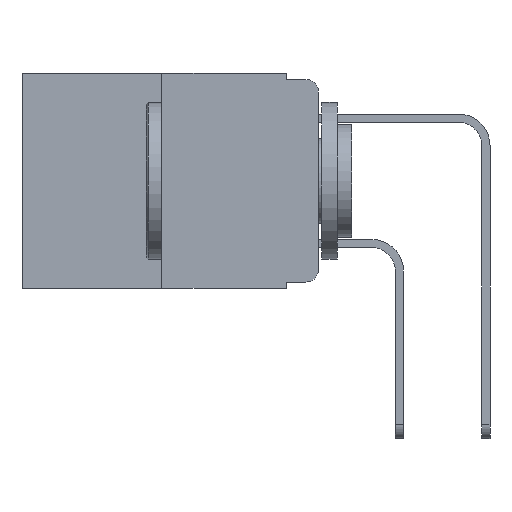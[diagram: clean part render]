
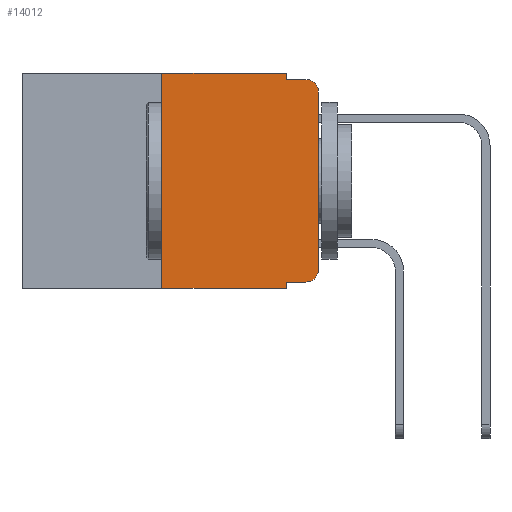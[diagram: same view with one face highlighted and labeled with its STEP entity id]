
A CAD part, left-side view. The second image highlights one B-rep face of the part: STEP entity #14012.
In plain terms, the highlighted planar face has unit normal (-1, 0, 0).
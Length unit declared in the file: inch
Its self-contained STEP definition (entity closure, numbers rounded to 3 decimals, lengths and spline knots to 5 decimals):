
#53 = DIRECTION ( 'NONE',  ( 0., -1., 0. ) ) ;
#161 = ORIENTED_EDGE ( 'NONE', *, *, #11742, .T. ) ;
#222 = VECTOR ( 'NONE', #8040, 39.37008 ) ;
#351 = CARTESIAN_POINT ( 'NONE',  ( 0., 0.051, -0.333 ) ) ;
#518 = ORIENTED_EDGE ( 'NONE', *, *, #749, .T. ) ;
#694 = ORIENTED_EDGE ( 'NONE', *, *, #9672, .F. ) ;
#749 = EDGE_CURVE ( 'NONE', #13618, #11591, #5216, .T. ) ;
#803 = CARTESIAN_POINT ( 'NONE',  ( 0., 0.02, -0.01 ) ) ;
#817 = CARTESIAN_POINT ( 'NONE',  ( 0., 0.473, 0. ) ) ;
#827 = CARTESIAN_POINT ( 'NONE',  ( 0., 0.25, 0. ) ) ;
#982 = VERTEX_POINT ( 'NONE', #7547 ) ;
#1018 = CARTESIAN_POINT ( 'NONE',  ( 0., 0.02, -0.333 ) ) ;
#1307 = VERTEX_POINT ( 'NONE', #3322 ) ;
#1341 = AXIS2_PLACEMENT_3D ( 'NONE', #12594, #12584, #11185 ) ;
#1362 = DIRECTION ( 'NONE',  ( 0., 0., 1. ) ) ;
#1385 = ORIENTED_EDGE ( 'NONE', *, *, #5163, .F. ) ;
#1508 = CARTESIAN_POINT ( 'NONE',  ( 0., 0.473, -0.343 ) ) ;
#1737 = CARTESIAN_POINT ( 'NONE',  ( 0., 0.051, -0.01 ) ) ;
#1792 = DIRECTION ( 'NONE',  ( 0., -1., 0. ) ) ;
#1810 = VERTEX_POINT ( 'NONE', #827 ) ;
#2152 = VERTEX_POINT ( 'NONE', #9073 ) ;
#2162 = CARTESIAN_POINT ( 'NONE',  ( 0., 0.25, -0.343 ) ) ;
#2793 = AXIS2_PLACEMENT_3D ( 'NONE', #12061, #5518, #13138 ) ;
#2830 = EDGE_CURVE ( 'NONE', #8331, #2152, #6092, .T. ) ;
#3057 = PLANE ( 'NONE',  #6744 ) ;
#3298 = ORIENTED_EDGE ( 'NONE', *, *, #7456, .F. ) ;
#3322 = CARTESIAN_POINT ( 'NONE',  ( 0., 0.051, -0.01 ) ) ;
#3576 = LINE ( 'NONE', #12252, #4311 ) ;
#3705 = VECTOR ( 'NONE', #7689, 39.37008 ) ;
#3823 = VECTOR ( 'NONE', #1792, 39.37008 ) ;
#4311 = VECTOR ( 'NONE', #6816, 39.37008 ) ;
#4470 = CARTESIAN_POINT ( 'NONE',  ( 0., 0.051, -0.333 ) ) ;
#4583 = VECTOR ( 'NONE', #4847, 39.37008 ) ;
#4745 = VERTEX_POINT ( 'NONE', #351 ) ;
#4847 = DIRECTION ( 'NONE',  ( 0., 0., -1. ) ) ;
#5006 = ORIENTED_EDGE ( 'NONE', *, *, #2830, .T. ) ;
#5163 = EDGE_CURVE ( 'NONE', #1810, #982, #13841, .T. ) ;
#5216 = CIRCLE ( 'NONE', #1341, 0.02 ) ;
#5259 = EDGE_CURVE ( 'NONE', #11591, #7807, #9276, .T. ) ;
#5347 = ORIENTED_EDGE ( 'NONE', *, *, #11361, .F. ) ;
#5518 = DIRECTION ( 'NONE',  ( -1., 0., 0. ) ) ;
#5609 = CARTESIAN_POINT ( 'NONE',  ( 0., 0., -0.03 ) ) ;
#5894 = CIRCLE ( 'NONE', #2793, 0.02 ) ;
#5976 = EDGE_CURVE ( 'NONE', #7807, #10627, #5894, .T. ) ;
#6092 = LINE ( 'NONE', #1508, #222 ) ;
#6336 = DIRECTION ( 'NONE',  ( 0., 0., -1. ) ) ;
#6744 = AXIS2_PLACEMENT_3D ( 'NONE', #817, #12872, #6336 ) ;
#6816 = DIRECTION ( 'NONE',  ( 0., 0., -1. ) ) ;
#7023 = VECTOR ( 'NONE', #1362, 39.37008 ) ;
#7105 = LINE ( 'NONE', #12445, #4583 ) ;
#7456 = EDGE_CURVE ( 'NONE', #1307, #10627, #13185, .T. ) ;
#7547 = CARTESIAN_POINT ( 'NONE',  ( 0., 0.051, 0. ) ) ;
#7626 = EDGE_CURVE ( 'NONE', #8331, #1810, #13339, .T. ) ;
#7689 = DIRECTION ( 'NONE',  ( 0., -1., 0. ) ) ;
#7807 = VERTEX_POINT ( 'NONE', #5609 ) ;
#7953 = CARTESIAN_POINT ( 'NONE',  ( 0., 0., 0. ) ) ;
#8040 = DIRECTION ( 'NONE',  ( 0., -1., 0. ) ) ;
#8078 = ORIENTED_EDGE ( 'NONE', *, *, #5259, .T. ) ;
#8331 = VERTEX_POINT ( 'NONE', #2162 ) ;
#8552 = EDGE_LOOP ( 'NONE', ( #8078, #14182, #3298, #694, #1385, #13009, #5006, #5347, #161, #518 ) ) ;
#8673 = CARTESIAN_POINT ( 'NONE',  ( 0., 0.25, 0. ) ) ;
#9073 = CARTESIAN_POINT ( 'NONE',  ( 0., 0.051, -0.343 ) ) ;
#9276 = LINE ( 'NONE', #7953, #7023 ) ;
#9672 = EDGE_CURVE ( 'NONE', #982, #1307, #3576, .T. ) ;
#9895 = CARTESIAN_POINT ( 'NONE',  ( 0., 0.473, 0. ) ) ;
#10283 = FACE_OUTER_BOUND ( 'NONE', #8552, .T. ) ;
#10471 = VECTOR ( 'NONE', #12953, 39.37008 ) ;
#10627 = VERTEX_POINT ( 'NONE', #803 ) ;
#10711 = LINE ( 'NONE', #4470, #3705 ) ;
#11185 = DIRECTION ( 'NONE',  ( 0., 0., -1. ) ) ;
#11361 = EDGE_CURVE ( 'NONE', #4745, #2152, #7105, .T. ) ;
#11591 = VERTEX_POINT ( 'NONE', #12887 ) ;
#11742 = EDGE_CURVE ( 'NONE', #4745, #13618, #10711, .T. ) ;
#12061 = CARTESIAN_POINT ( 'NONE',  ( 0., 0.02, -0.03 ) ) ;
#12252 = CARTESIAN_POINT ( 'NONE',  ( 0., 0.051, 0. ) ) ;
#12445 = CARTESIAN_POINT ( 'NONE',  ( 0., 0.051, 0. ) ) ;
#12584 = DIRECTION ( 'NONE',  ( -1., 0., 0. ) ) ;
#12594 = CARTESIAN_POINT ( 'NONE',  ( 0., 0.02, -0.313 ) ) ;
#12872 = DIRECTION ( 'NONE',  ( 1., 0., 0. ) ) ;
#12887 = CARTESIAN_POINT ( 'NONE',  ( 0., 0., -0.313 ) ) ;
#12953 = DIRECTION ( 'NONE',  ( 0., 0., 1. ) ) ;
#13009 = ORIENTED_EDGE ( 'NONE', *, *, #7626, .F. ) ;
#13138 = DIRECTION ( 'NONE',  ( 0., 0., -1. ) ) ;
#13185 = LINE ( 'NONE', #1737, #3823 ) ;
#13339 = LINE ( 'NONE', #8673, #10471 ) ;
#13501 = VECTOR ( 'NONE', #53, 39.37008 ) ;
#13618 = VERTEX_POINT ( 'NONE', #1018 ) ;
#13841 = LINE ( 'NONE', #9895, #13501 ) ;
#14012 = ADVANCED_FACE ( 'NONE', ( #10283 ), #3057, .F. ) ;
#14182 = ORIENTED_EDGE ( 'NONE', *, *, #5976, .T. ) ;
